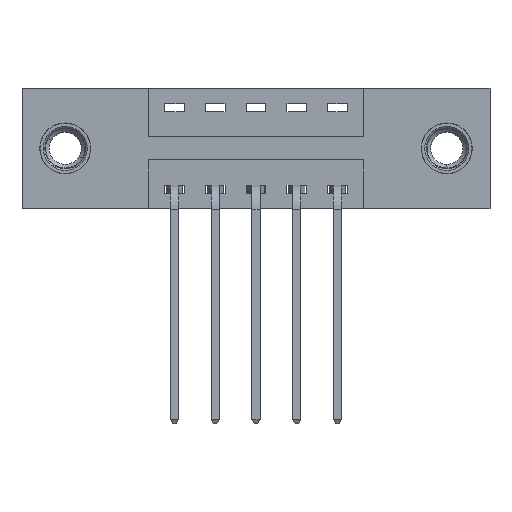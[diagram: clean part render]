
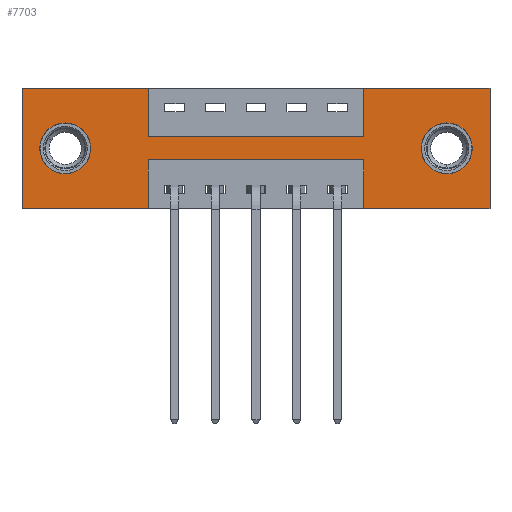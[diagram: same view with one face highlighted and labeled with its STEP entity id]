
A CAD part, front view. The second image highlights one B-rep face of the part: STEP entity #7703.
In plain terms, the highlighted planar face has unit normal (0, -1, 0).
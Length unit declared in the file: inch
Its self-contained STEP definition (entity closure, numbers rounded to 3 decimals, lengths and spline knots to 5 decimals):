
#51 = VERTEX_POINT ( 'NONE', #1276 ) ;
#95 = VERTEX_POINT ( 'NONE', #3619 ) ;
#297 = CARTESIAN_POINT ( 'NONE',  ( 0.3875, 0., -0.15 ) ) ;
#312 = VERTEX_POINT ( 'NONE', #3044 ) ;
#629 = VERTEX_POINT ( 'NONE', #4836 ) ;
#640 = CARTESIAN_POINT ( 'NONE',  ( 1.3025, 0., -0.263 ) ) ;
#645 = ORIENTED_EDGE ( 'NONE', *, *, #4120, .T. ) ;
#670 = ORIENTED_EDGE ( 'NONE', *, *, #7775, .T. ) ;
#768 = ORIENTED_EDGE ( 'NONE', *, *, #5602, .T. ) ;
#774 = VERTEX_POINT ( 'NONE', #7752 ) ;
#928 = ORIENTED_EDGE ( 'NONE', *, *, #2415, .T. ) ;
#937 = CARTESIAN_POINT ( 'NONE',  ( 1.0475, 0., -0.22 ) ) ;
#959 = LINE ( 'NONE', #8743, #2634 ) ;
#983 = AXIS2_PLACEMENT_3D ( 'NONE', #8599, #2400, #7279 ) ;
#1082 = VERTEX_POINT ( 'NONE', #2422 ) ;
#1167 = ORIENTED_EDGE ( 'NONE', *, *, #3316, .F. ) ;
#1238 = ORIENTED_EDGE ( 'NONE', *, *, #4102, .F. ) ;
#1276 = CARTESIAN_POINT ( 'NONE',  ( 0.1325, 0., -0.263 ) ) ;
#1487 = ORIENTED_EDGE ( 'NONE', *, *, #7764, .F. ) ;
#1496 = ORIENTED_EDGE ( 'NONE', *, *, #4239, .F. ) ;
#1539 = AXIS2_PLACEMENT_3D ( 'NONE', #8046, #3929, #8716 ) ;
#1594 = ORIENTED_EDGE ( 'NONE', *, *, #5890, .F. ) ;
#1663 = DIRECTION ( 'NONE',  ( 0., 0., -1. ) ) ;
#1695 = ORIENTED_EDGE ( 'NONE', *, *, #5076, .F. ) ;
#1713 = DIRECTION ( 'NONE',  ( 1., 0., 0. ) ) ;
#1879 = ORIENTED_EDGE ( 'NONE', *, *, #9181, .F. ) ;
#1887 = ORIENTED_EDGE ( 'NONE', *, *, #7986, .F. ) ;
#1969 = VERTEX_POINT ( 'NONE', #8280 ) ;
#1974 = LINE ( 'NONE', #6669, #5311 ) ;
#1978 = ORIENTED_EDGE ( 'NONE', *, *, #8552, .F. ) ;
#2001 = ORIENTED_EDGE ( 'NONE', *, *, #2701, .F. ) ;
#2018 = ORIENTED_EDGE ( 'NONE', *, *, #5104, .F. ) ;
#2032 = CARTESIAN_POINT ( 'NONE',  ( 0.1325, 0., -0.185 ) ) ;
#2108 = ORIENTED_EDGE ( 'NONE', *, *, #7911, .F. ) ;
#2156 = DIRECTION ( 'NONE',  ( -1., 0., 0. ) ) ;
#2209 = EDGE_LOOP ( 'NONE', ( #645, #670 ) ) ;
#2257 = FACE_OUTER_BOUND ( 'NONE', #7621, .T. ) ;
#2400 = DIRECTION ( 'NONE',  ( 0., -1., 0. ) ) ;
#2415 = EDGE_CURVE ( 'NONE', #51, #1969, #7459, .T. ) ;
#2422 = CARTESIAN_POINT ( 'NONE',  ( 0.3875, 0., -0.15 ) ) ;
#2530 = VERTEX_POINT ( 'NONE', #4426 ) ;
#2619 = CARTESIAN_POINT ( 'NONE',  ( 0.3875, 0., 0. ) ) ;
#2634 = VECTOR ( 'NONE', #3993, 39.37008 ) ;
#2662 = DIRECTION ( 'NONE',  ( -1., 0., 0. ) ) ;
#2701 = EDGE_CURVE ( 'NONE', #774, #6742, #8910, .T. ) ;
#2803 = DIRECTION ( 'NONE',  ( 0., 1., 0. ) ) ;
#2817 = DIRECTION ( 'NONE',  ( 0., 0., 1. ) ) ;
#2900 = CARTESIAN_POINT ( 'NONE',  ( 0., 0., -0.37 ) ) ;
#3044 = CARTESIAN_POINT ( 'NONE',  ( 0.3875, 0., -0.22 ) ) ;
#3090 = VECTOR ( 'NONE', #2156, 39.37008 ) ;
#3129 = DIRECTION ( 'NONE',  ( 0., 0., -1. ) ) ;
#3167 = CARTESIAN_POINT ( 'NONE',  ( 0.3875, 0., -0.37 ) ) ;
#3185 = VERTEX_POINT ( 'NONE', #4413 ) ;
#3259 = CARTESIAN_POINT ( 'NONE',  ( 0., 0., 0. ) ) ;
#3306 = CIRCLE ( 'NONE', #1539, 0.078 ) ;
#3316 = EDGE_CURVE ( 'NONE', #312, #3842, #9186, .T. ) ;
#3398 = CARTESIAN_POINT ( 'NONE',  ( 0., 0., -0.37 ) ) ;
#3401 = DIRECTION ( 'NONE',  ( 0., 0., 1. ) ) ;
#3441 = VERTEX_POINT ( 'NONE', #937 ) ;
#3450 = AXIS2_PLACEMENT_3D ( 'NONE', #8804, #6135, #3495 ) ;
#3495 = DIRECTION ( 'NONE',  ( 0., 0., 1. ) ) ;
#3619 = CARTESIAN_POINT ( 'NONE',  ( 1.435, 0., 0. ) ) ;
#3842 = VERTEX_POINT ( 'NONE', #6003 ) ;
#3886 = CARTESIAN_POINT ( 'NONE',  ( 0., 0., 0. ) ) ;
#3929 = DIRECTION ( 'NONE',  ( 0., 1., 0. ) ) ;
#3993 = DIRECTION ( 'NONE',  ( 0., 0., 1. ) ) ;
#4064 = LINE ( 'NONE', #4769, #7511 ) ;
#4102 = EDGE_CURVE ( 'NONE', #3441, #312, #8061, .T. ) ;
#4120 = EDGE_CURVE ( 'NONE', #629, #4372, #6026, .T. ) ;
#4239 = EDGE_CURVE ( 'NONE', #6308, #3185, #4941, .T. ) ;
#4372 = VERTEX_POINT ( 'NONE', #640 ) ;
#4413 = CARTESIAN_POINT ( 'NONE',  ( 1.0475, 0., -0.37 ) ) ;
#4426 = CARTESIAN_POINT ( 'NONE',  ( 1.0475, 0., 0. ) ) ;
#4646 = VERTEX_POINT ( 'NONE', #3398 ) ;
#4769 = CARTESIAN_POINT ( 'NONE',  ( 0., 0., -0.37 ) ) ;
#4836 = CARTESIAN_POINT ( 'NONE',  ( 1.3025, 0., -0.107 ) ) ;
#4856 = CARTESIAN_POINT ( 'NONE',  ( 0.3875, 0., -0.22 ) ) ;
#4926 = LINE ( 'NONE', #3259, #6771 ) ;
#4941 = LINE ( 'NONE', #2900, #3090 ) ;
#5076 = EDGE_CURVE ( 'NONE', #2530, #95, #4926, .T. ) ;
#5104 = EDGE_CURVE ( 'NONE', #4646, #774, #959, .T. ) ;
#5122 = VECTOR ( 'NONE', #5936, 39.37008 ) ;
#5249 = DIRECTION ( 'NONE',  ( 1., 0., 0. ) ) ;
#5311 = VECTOR ( 'NONE', #1663, 39.37008 ) ;
#5401 = AXIS2_PLACEMENT_3D ( 'NONE', #2032, #6979, #2817 ) ;
#5404 = VECTOR ( 'NONE', #3401, 39.37008 ) ;
#5425 = CARTESIAN_POINT ( 'NONE',  ( 1.0475, 0., 0. ) ) ;
#5516 = DIRECTION ( 'NONE',  ( -1., 0., 0. ) ) ;
#5521 = CARTESIAN_POINT ( 'NONE',  ( 1.435, 0., -0.37 ) ) ;
#5599 = EDGE_LOOP ( 'NONE', ( #768, #928 ) ) ;
#5602 = EDGE_CURVE ( 'NONE', #1969, #51, #9250, .T. ) ;
#5762 = FACE_BOUND ( 'NONE', #2209, .T. ) ;
#5890 = EDGE_CURVE ( 'NONE', #95, #6308, #6963, .T. ) ;
#5936 = DIRECTION ( 'NONE',  ( 0., 0., 1. ) ) ;
#6003 = CARTESIAN_POINT ( 'NONE',  ( 0.3875, 0., -0.37 ) ) ;
#6004 = FACE_BOUND ( 'NONE', #5599, .T. ) ;
#6026 = CIRCLE ( 'NONE', #6288, 0.078 ) ;
#6135 = DIRECTION ( 'NONE',  ( 0., 1., 0. ) ) ;
#6288 = AXIS2_PLACEMENT_3D ( 'NONE', #6968, #2803, #7646 ) ;
#6308 = VERTEX_POINT ( 'NONE', #5521 ) ;
#6582 = PLANE ( 'NONE',  #983 ) ;
#6650 = CARTESIAN_POINT ( 'NONE',  ( 1.0475, 0., -0.37 ) ) ;
#6669 = CARTESIAN_POINT ( 'NONE',  ( 0.3875, 0., 0. ) ) ;
#6694 = VERTEX_POINT ( 'NONE', #8085 ) ;
#6742 = VERTEX_POINT ( 'NONE', #2619 ) ;
#6771 = VECTOR ( 'NONE', #1713, 39.37008 ) ;
#6868 = LINE ( 'NONE', #297, #8664 ) ;
#6899 = VECTOR ( 'NONE', #5516, 39.37008 ) ;
#6963 = LINE ( 'NONE', #7957, #8546 ) ;
#6968 = CARTESIAN_POINT ( 'NONE',  ( 1.3025, 0., -0.185 ) ) ;
#6979 = DIRECTION ( 'NONE',  ( 0., 1., 0. ) ) ;
#7131 = VECTOR ( 'NONE', #5249, 39.37008 ) ;
#7226 = VECTOR ( 'NONE', #7311, 39.37008 ) ;
#7266 = LINE ( 'NONE', #5425, #5404 ) ;
#7279 = DIRECTION ( 'NONE',  ( 0., 0., -1. ) ) ;
#7311 = DIRECTION ( 'NONE',  ( 0., 0., -1. ) ) ;
#7459 = CIRCLE ( 'NONE', #3450, 0.078 ) ;
#7511 = VECTOR ( 'NONE', #2662, 39.37008 ) ;
#7621 = EDGE_LOOP ( 'NONE', ( #1167, #1238, #1487, #1496, #1594, #1695, #1879, #1887, #1978, #2001, #2018, #2108 ) ) ;
#7646 = DIRECTION ( 'NONE',  ( 0., 0., -1. ) ) ;
#7703 = ADVANCED_FACE ( 'NONE', ( #5762, #6004, #2257 ), #6582, .T. ) ;
#7752 = CARTESIAN_POINT ( 'NONE',  ( 0., 0., 0. ) ) ;
#7764 = EDGE_CURVE ( 'NONE', #3185, #3441, #8967, .T. ) ;
#7775 = EDGE_CURVE ( 'NONE', #4372, #629, #3306, .T. ) ;
#7911 = EDGE_CURVE ( 'NONE', #3842, #4646, #4064, .T. ) ;
#7957 = CARTESIAN_POINT ( 'NONE',  ( 1.435, 0., 0. ) ) ;
#7986 = EDGE_CURVE ( 'NONE', #1082, #6694, #6868, .T. ) ;
#8046 = CARTESIAN_POINT ( 'NONE',  ( 1.3025, 0., -0.185 ) ) ;
#8061 = LINE ( 'NONE', #4856, #6899 ) ;
#8085 = CARTESIAN_POINT ( 'NONE',  ( 1.0475, 0., -0.15 ) ) ;
#8280 = CARTESIAN_POINT ( 'NONE',  ( 0.1325, 0., -0.107 ) ) ;
#8293 = DIRECTION ( 'NONE',  ( 1., 0., 0. ) ) ;
#8546 = VECTOR ( 'NONE', #3129, 39.37008 ) ;
#8552 = EDGE_CURVE ( 'NONE', #6742, #1082, #1974, .T. ) ;
#8599 = CARTESIAN_POINT ( 'NONE',  ( 0., 0., -0.37 ) ) ;
#8664 = VECTOR ( 'NONE', #8293, 39.37008 ) ;
#8716 = DIRECTION ( 'NONE',  ( 0., 0., -1. ) ) ;
#8743 = CARTESIAN_POINT ( 'NONE',  ( 0., 0., 0. ) ) ;
#8804 = CARTESIAN_POINT ( 'NONE',  ( 0.1325, 0., -0.185 ) ) ;
#8910 = LINE ( 'NONE', #3886, #7131 ) ;
#8967 = LINE ( 'NONE', #6650, #5122 ) ;
#9181 = EDGE_CURVE ( 'NONE', #6694, #2530, #7266, .T. ) ;
#9186 = LINE ( 'NONE', #3167, #7226 ) ;
#9250 = CIRCLE ( 'NONE', #5401, 0.078 ) ;
